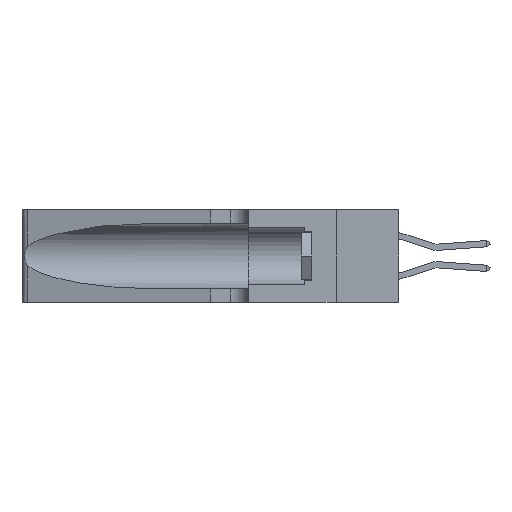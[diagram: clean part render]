
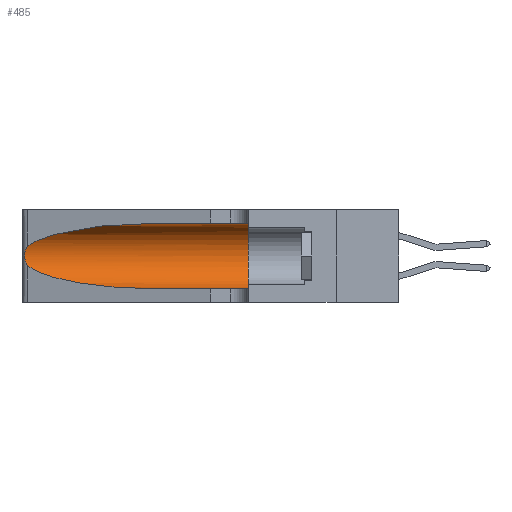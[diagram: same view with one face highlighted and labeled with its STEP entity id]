
A CAD part, left-side view. The second image highlights one B-rep face of the part: STEP entity #485.
In plain terms, the highlighted cylindrical face has radius 3.308 mm (diameter 6.617 mm), a partial arc.
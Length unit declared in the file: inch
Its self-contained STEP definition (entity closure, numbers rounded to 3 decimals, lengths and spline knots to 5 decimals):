
#10 =( BOUNDED_CURVE ( )  B_SPLINE_CURVE ( 3, ( #11178, #25919, #7233, #19046 ),
 .UNSPECIFIED., .F., .F. ) 
 B_SPLINE_CURVE_WITH_KNOTS ( ( 4, 4 ),
 ( 3.44316, 4.71239 ),
 .UNSPECIFIED. ) 
 CURVE ( )  GEOMETRIC_REPRESENTATION_ITEM ( )  RATIONAL_B_SPLINE_CURVE ( ( 1., 0.87, 0.87, 1. ) ) 
 REPRESENTATION_ITEM ( '' )  );
#485 = ADVANCED_FACE ( 'NONE', ( #18706 ), #24715, .F. ) ;
#1600 = VECTOR ( 'NONE', #6533, 39.37008 ) ;
#2259 = CARTESIAN_POINT ( 'NONE',  ( 0.25555, 1.22994, 0.2215 ) ) ;
#2902 = DIRECTION ( 'NONE',  ( 0., 1., 0. ) ) ;
#3004 = EDGE_CURVE ( 'NONE', #9803, #30111, #10205, .T. ) ;
#4220 =( BOUNDED_CURVE ( )  B_SPLINE_CURVE ( 3, ( #10774, #17637, #17739, #5668 ),
 .UNSPECIFIED., .F., .F. ) 
 B_SPLINE_CURVE_WITH_KNOTS ( ( 4, 4 ),
 ( 1.5708, 2.84003 ),
 .UNSPECIFIED. ) 
 CURVE ( )  GEOMETRIC_REPRESENTATION_ITEM ( )  RATIONAL_B_SPLINE_CURVE ( ( 1., 0.87, 0.87, 1. ) ) 
 REPRESENTATION_ITEM ( '' )  );
#4255 = CARTESIAN_POINT ( 'NONE',  ( 0.25787, 1.23484, 0.2124 ) ) ;
#5038 = ORIENTED_EDGE ( 'NONE', *, *, #26730, .T. ) ;
#5258 = AXIS2_PLACEMENT_3D ( 'NONE', #25887, #13773, #23964 ) ;
#5668 = CARTESIAN_POINT ( 'NONE',  ( 0.25487, 1.22718, 0.22369 ) ) ;
#5697 = CARTESIAN_POINT ( 'NONE',  ( 0.25639, 1.23186, 0.15144 ) ) ;
#5740 = AXIS2_PLACEMENT_3D ( 'NONE', #17405, #2902, #7871 ) ;
#6533 = DIRECTION ( 'NONE',  ( 0., -1., 0. ) ) ;
#7232 = VERTEX_POINT ( 'NONE', #22212 ) ;
#7233 = CARTESIAN_POINT ( 'NONE',  ( 0.18966, 0.96281, 0.05475 ) ) ;
#7453 = CARTESIAN_POINT ( 'NONE',  ( 0.1305, 1.61858, 0.05475 ) ) ;
#7871 = DIRECTION ( 'NONE',  ( 0., 0., 1. ) ) ;
#8763 = CARTESIAN_POINT ( 'NONE',  ( 0.25487, 1.22718, 0.22369 ) ) ;
#8773 = VECTOR ( 'NONE', #24425, 39.37008 ) ;
#9803 = VERTEX_POINT ( 'NONE', #25688 ) ;
#10205 = CIRCLE ( 'NONE', #5740, 0.13025 ) ;
#10259 = CARTESIAN_POINT ( 'NONE',  ( 0.25789, 1.23486, 0.15765 ) ) ;
#10774 = CARTESIAN_POINT ( 'NONE',  ( 0.1305, 0.72297, 0.31525 ) ) ;
#11178 = CARTESIAN_POINT ( 'NONE',  ( 0.25487, 1.22718, 0.14631 ) ) ;
#12086 = CARTESIAN_POINT ( 'NONE',  ( 0.26075, 1.23896, 0.178 ) ) ;
#12280 = CARTESIAN_POINT ( 'NONE',  ( 0.25854, 1.2359, 0.20912 ) ) ;
#13773 = DIRECTION ( 'NONE',  ( 0., -1., 0. ) ) ;
#14809 = VERTEX_POINT ( 'NONE', #8763 ) ;
#16602 = EDGE_CURVE ( 'NONE', #7232, #9803, #29223, .T. ) ;
#17061 = EDGE_LOOP ( 'NONE', ( #5038, #28814, #17176, #29792, #26213, #20744 ) ) ;
#17176 = ORIENTED_EDGE ( 'NONE', *, *, #22003, .T. ) ;
#17339 = CARTESIAN_POINT ( 'NONE',  ( 0.25555, 1.22993, 0.14849 ) ) ;
#17405 = CARTESIAN_POINT ( 'NONE',  ( 0.1305, 0.35, 0.185 ) ) ;
#17637 = CARTESIAN_POINT ( 'NONE',  ( 0.18966, 0.96281, 0.31525 ) ) ;
#17739 = CARTESIAN_POINT ( 'NONE',  ( 0.2373, 1.15595, 0.28018 ) ) ;
#18706 = FACE_OUTER_BOUND ( 'NONE', #17061, .T. ) ;
#18812 = CARTESIAN_POINT ( 'NONE',  ( 0.25639, 1.23184, 0.21858 ) ) ;
#18941 = CARTESIAN_POINT ( 'NONE',  ( 0.1305, 1.61858, 0.31525 ) ) ;
#19046 = CARTESIAN_POINT ( 'NONE',  ( 0.1305, 0.72297, 0.05475 ) ) ;
#20744 = ORIENTED_EDGE ( 'NONE', *, *, #16602, .F. ) ;
#21552 = B_SPLINE_CURVE_WITH_KNOTS ( 'NONE', 3,
 ( #31277, #2259, #18812, #4255, #12280, #22040, #29145, #12086, #26906, #21758, #10259, #5697, #17339, #27431 ),
 .UNSPECIFIED., .F., .F.,
 ( 4, 2, 2, 2, 2, 2, 4 ),
 ( 0., 0.00027, 0.00053, 0.00107, 0.0016, 0.00187, 0.00214 ),
 .UNSPECIFIED. ) ;
#21758 = CARTESIAN_POINT ( 'NONE',  ( 0.25856, 1.23593, 0.16098 ) ) ;
#22003 = EDGE_CURVE ( 'NONE', #27544, #29837, #10, .T. ) ;
#22040 = CARTESIAN_POINT ( 'NONE',  ( 0.26018, 1.23835, 0.19895 ) ) ;
#22212 = CARTESIAN_POINT ( 'NONE',  ( 0.1305, 0.72297, 0.31525 ) ) ;
#22450 = CARTESIAN_POINT ( 'NONE',  ( 0.1305, 0.35, 0.05475 ) ) ;
#23130 = EDGE_CURVE ( 'NONE', #14809, #27544, #21552, .T. ) ;
#23964 = DIRECTION ( 'NONE',  ( 0., 0., -1. ) ) ;
#24425 = DIRECTION ( 'NONE',  ( 0., -1., 0. ) ) ;
#24715 = CYLINDRICAL_SURFACE ( 'NONE', #5258, 0.13025 ) ;
#25688 = CARTESIAN_POINT ( 'NONE',  ( 0.1305, 0.35, 0.31525 ) ) ;
#25887 = CARTESIAN_POINT ( 'NONE',  ( 0.1305, 1.61858, 0.185 ) ) ;
#25919 = CARTESIAN_POINT ( 'NONE',  ( 0.2373, 1.15595, 0.08982 ) ) ;
#26213 = ORIENTED_EDGE ( 'NONE', *, *, #3004, .F. ) ;
#26730 = EDGE_CURVE ( 'NONE', #7232, #14809, #4220, .T. ) ;
#26906 = CARTESIAN_POINT ( 'NONE',  ( 0.26017, 1.23833, 0.17102 ) ) ;
#27083 = CARTESIAN_POINT ( 'NONE',  ( 0.1305, 0.72297, 0.05475 ) ) ;
#27431 = CARTESIAN_POINT ( 'NONE',  ( 0.25487, 1.22718, 0.14631 ) ) ;
#27544 = VERTEX_POINT ( 'NONE', #31305 ) ;
#28706 = EDGE_CURVE ( 'NONE', #29837, #30111, #30744, .T. ) ;
#28814 = ORIENTED_EDGE ( 'NONE', *, *, #23130, .T. ) ;
#29145 = CARTESIAN_POINT ( 'NONE',  ( 0.26075, 1.23896, 0.19203 ) ) ;
#29223 = LINE ( 'NONE', #18941, #1600 ) ;
#29792 = ORIENTED_EDGE ( 'NONE', *, *, #28706, .T. ) ;
#29837 = VERTEX_POINT ( 'NONE', #27083 ) ;
#30111 = VERTEX_POINT ( 'NONE', #22450 ) ;
#30744 = LINE ( 'NONE', #7453, #8773 ) ;
#31277 = CARTESIAN_POINT ( 'NONE',  ( 0.25487, 1.22718, 0.22369 ) ) ;
#31305 = CARTESIAN_POINT ( 'NONE',  ( 0.25487, 1.22718, 0.14631 ) ) ;
